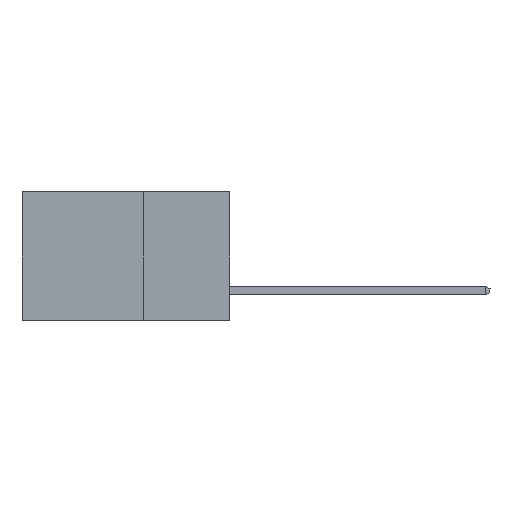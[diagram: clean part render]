
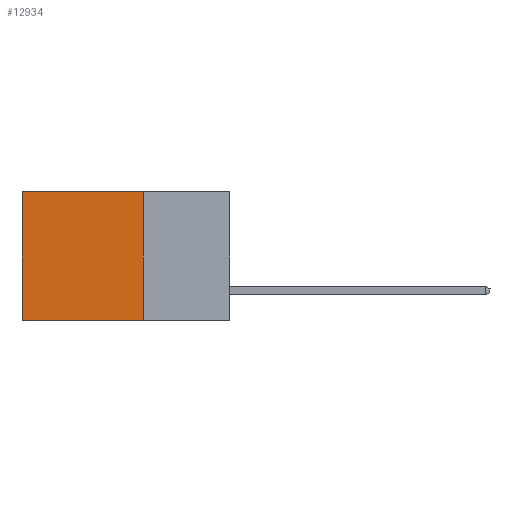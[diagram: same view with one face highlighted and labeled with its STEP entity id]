
A CAD part, left-side view. The second image highlights one B-rep face of the part: STEP entity #12934.
In plain terms, the highlighted planar face has unit normal (-1, 0, 0).
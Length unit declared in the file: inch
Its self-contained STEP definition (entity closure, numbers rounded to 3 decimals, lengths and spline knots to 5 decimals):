
#871 = ORIENTED_EDGE ( 'NONE', *, *, #6454, .F. ) ;
#2059 = DIRECTION ( 'NONE',  ( 0., 0., -1. ) ) ;
#2436 = PLANE ( 'NONE',  #17963 ) ;
#2509 = LINE ( 'NONE', #8159, #23185 ) ;
#2933 = CARTESIAN_POINT ( 'NONE',  ( 0.2615, 0.6, -0.37 ) ) ;
#3279 = VECTOR ( 'NONE', #12348, 39.37008 ) ;
#3734 = VECTOR ( 'NONE', #13974, 39.37008 ) ;
#4228 = CARTESIAN_POINT ( 'NONE',  ( 0.2615, 0.25, -0.37 ) ) ;
#6353 = VERTEX_POINT ( 'NONE', #19139 ) ;
#6454 = EDGE_CURVE ( 'NONE', #14088, #9084, #17875, .T. ) ;
#6932 = ORIENTED_EDGE ( 'NONE', *, *, #18015, .F. ) ;
#8159 = CARTESIAN_POINT ( 'NONE',  ( 0.2615, 0.25, 0. ) ) ;
#8472 = CARTESIAN_POINT ( 'NONE',  ( 0.2615, 0.6, -0.37 ) ) ;
#9084 = VERTEX_POINT ( 'NONE', #8472 ) ;
#11090 = ORIENTED_EDGE ( 'NONE', *, *, #14477, .T. ) ;
#11819 = CARTESIAN_POINT ( 'NONE',  ( 0.2615, 0.25, -0.37 ) ) ;
#12213 = EDGE_LOOP ( 'NONE', ( #15828, #871, #6932, #11090 ) ) ;
#12348 = DIRECTION ( 'NONE',  ( 0., 0., -1. ) ) ;
#12934 = ADVANCED_FACE ( 'NONE', ( #15465 ), #2436, .F. ) ;
#13083 = CARTESIAN_POINT ( 'NONE',  ( 0.2615, 0.25, -0.37 ) ) ;
#13188 = CARTESIAN_POINT ( 'NONE',  ( 0.2615, 0.6, 0. ) ) ;
#13840 = DIRECTION ( 'NONE',  ( 1., 0., 0. ) ) ;
#13974 = DIRECTION ( 'NONE',  ( 0., 0., -1. ) ) ;
#14088 = VERTEX_POINT ( 'NONE', #13083 ) ;
#14477 = EDGE_CURVE ( 'NONE', #6353, #19645, #2509, .T. ) ;
#15465 = FACE_OUTER_BOUND ( 'NONE', #12213, .T. ) ;
#15828 = ORIENTED_EDGE ( 'NONE', *, *, #19404, .T. ) ;
#15999 = LINE ( 'NONE', #4228, #3279 ) ;
#16216 = LINE ( 'NONE', #2933, #3734 ) ;
#17753 = DIRECTION ( 'NONE',  ( 0., 1., 0. ) ) ;
#17875 = LINE ( 'NONE', #21760, #19151 ) ;
#17963 = AXIS2_PLACEMENT_3D ( 'NONE', #11819, #13840, #2059 ) ;
#18015 = EDGE_CURVE ( 'NONE', #6353, #14088, #15999, .T. ) ;
#19139 = CARTESIAN_POINT ( 'NONE',  ( 0.2615, 0.25, 0. ) ) ;
#19151 = VECTOR ( 'NONE', #17753, 39.37008 ) ;
#19404 = EDGE_CURVE ( 'NONE', #19645, #9084, #16216, .T. ) ;
#19645 = VERTEX_POINT ( 'NONE', #13188 ) ;
#21760 = CARTESIAN_POINT ( 'NONE',  ( 0.2615, 0.25, -0.37 ) ) ;
#23185 = VECTOR ( 'NONE', #23426, 39.37008 ) ;
#23426 = DIRECTION ( 'NONE',  ( 0., 1., 0. ) ) ;
